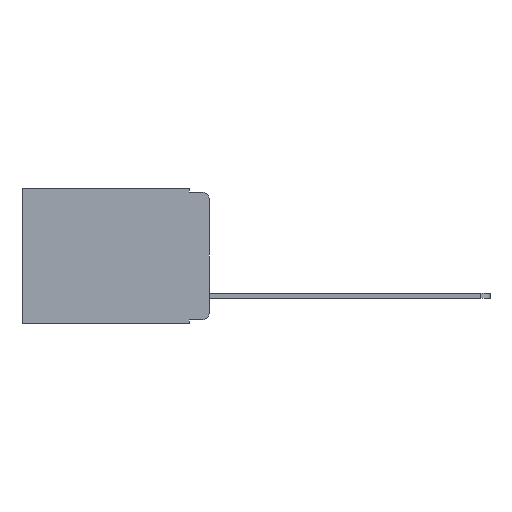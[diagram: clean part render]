
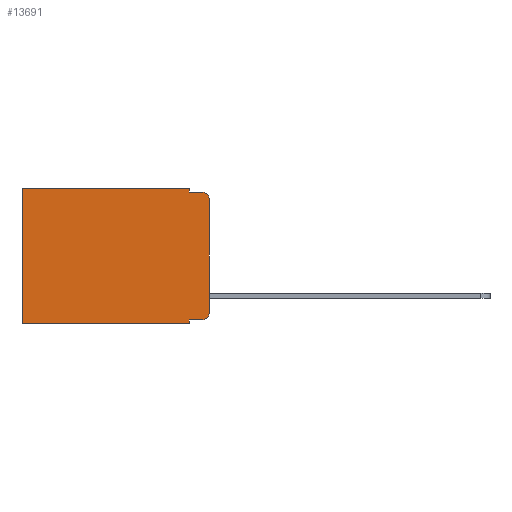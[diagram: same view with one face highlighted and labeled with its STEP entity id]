
A CAD part, left-side view. The second image highlights one B-rep face of the part: STEP entity #13691.
In plain terms, the highlighted planar face has unit normal (-1, 0, 0).
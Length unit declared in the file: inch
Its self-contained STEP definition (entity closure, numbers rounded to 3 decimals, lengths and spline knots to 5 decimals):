
#201 = DIRECTION ( 'NONE',  ( 0., 1., 0. ) ) ;
#272 = ORIENTED_EDGE ( 'NONE', *, *, #9066, .F. ) ;
#332 = CIRCLE ( 'NONE', #11500, 0.02 ) ;
#483 = ORIENTED_EDGE ( 'NONE', *, *, #6219, .T. ) ;
#559 = DIRECTION ( 'NONE',  ( 0., 0., -1. ) ) ;
#940 = CARTESIAN_POINT ( 'NONE',  ( 0.298, 0.051, -0.333 ) ) ;
#956 = CARTESIAN_POINT ( 'NONE',  ( 0.298, 0.051, 0. ) ) ;
#1117 = ORIENTED_EDGE ( 'NONE', *, *, #10961, .T. ) ;
#1229 = EDGE_CURVE ( 'NONE', #6926, #6484, #13971, .T. ) ;
#1267 = ORIENTED_EDGE ( 'NONE', *, *, #7857, .F. ) ;
#1395 = LINE ( 'NONE', #8242, #12024 ) ;
#1463 = VERTEX_POINT ( 'NONE', #2653 ) ;
#1621 = CARTESIAN_POINT ( 'NONE',  ( 0.298, 0., 0. ) ) ;
#1997 = CARTESIAN_POINT ( 'NONE',  ( 0.298, 0.473, 0. ) ) ;
#2028 = EDGE_LOOP ( 'NONE', ( #5095, #5801, #4200, #4830, #11334, #1117, #272, #1267, #5888, #483 ) ) ;
#2122 = VERTEX_POINT ( 'NONE', #2125 ) ;
#2125 = CARTESIAN_POINT ( 'NONE',  ( 0.298, 0., -0.03 ) ) ;
#2170 = VERTEX_POINT ( 'NONE', #4646 ) ;
#2208 = AXIS2_PLACEMENT_3D ( 'NONE', #11327, #4091, #12446 ) ;
#2275 = CARTESIAN_POINT ( 'NONE',  ( 0.298, 0.051, 0. ) ) ;
#2415 = LINE ( 'NONE', #15195, #8779 ) ;
#2466 = VECTOR ( 'NONE', #9824, 39.37008 ) ;
#2653 = CARTESIAN_POINT ( 'NONE',  ( 0.298, 0., -0.313 ) ) ;
#2771 = VERTEX_POINT ( 'NONE', #940 ) ;
#3162 = LINE ( 'NONE', #1621, #15330 ) ;
#4059 = VERTEX_POINT ( 'NONE', #7688 ) ;
#4091 = DIRECTION ( 'NONE',  ( -1., 0., 0. ) ) ;
#4178 = VERTEX_POINT ( 'NONE', #11527 ) ;
#4200 = ORIENTED_EDGE ( 'NONE', *, *, #12445, .F. ) ;
#4646 = CARTESIAN_POINT ( 'NONE',  ( 0.298, 0.02, -0.333 ) ) ;
#4824 = VECTOR ( 'NONE', #5585, 39.37008 ) ;
#4830 = ORIENTED_EDGE ( 'NONE', *, *, #11712, .F. ) ;
#4831 = LINE ( 'NONE', #1997, #14506 ) ;
#5095 = ORIENTED_EDGE ( 'NONE', *, *, #11428, .F. ) ;
#5585 = DIRECTION ( 'NONE',  ( 0., -1., 0. ) ) ;
#5801 = ORIENTED_EDGE ( 'NONE', *, *, #14666, .T. ) ;
#5848 = PLANE ( 'NONE',  #13890 ) ;
#5888 = ORIENTED_EDGE ( 'NONE', *, *, #7023, .T. ) ;
#5904 = CARTESIAN_POINT ( 'NONE',  ( 0.298, 0., 0. ) ) ;
#5924 = VERTEX_POINT ( 'NONE', #10656 ) ;
#6032 = VECTOR ( 'NONE', #12068, 39.37008 ) ;
#6219 = EDGE_CURVE ( 'NONE', #2170, #1463, #332, .T. ) ;
#6484 = VERTEX_POINT ( 'NONE', #10103 ) ;
#6793 = LINE ( 'NONE', #956, #6032 ) ;
#6926 = VERTEX_POINT ( 'NONE', #10390 ) ;
#7023 = EDGE_CURVE ( 'NONE', #2771, #2170, #1395, .T. ) ;
#7277 = DIRECTION ( 'NONE',  ( 0., 1., 0. ) ) ;
#7688 = CARTESIAN_POINT ( 'NONE',  ( 0.298, 0.02, -0.01 ) ) ;
#7776 = CARTESIAN_POINT ( 'NONE',  ( 0.298, 0.02, -0.313 ) ) ;
#7857 = EDGE_CURVE ( 'NONE', #2771, #14111, #11846, .T. ) ;
#8067 = DIRECTION ( 'NONE',  ( 0., 0., -1. ) ) ;
#8242 = CARTESIAN_POINT ( 'NONE',  ( 0.298, 0.051, -0.333 ) ) ;
#8344 = DIRECTION ( 'NONE',  ( 1., 0., 0. ) ) ;
#8779 = VECTOR ( 'NONE', #7277, 39.37008 ) ;
#9066 = EDGE_CURVE ( 'NONE', #14111, #4178, #2415, .T. ) ;
#9176 = CARTESIAN_POINT ( 'NONE',  ( 0.298, 0.051, -0.01 ) ) ;
#9586 = DIRECTION ( 'NONE',  ( 0., 0., -1. ) ) ;
#9824 = DIRECTION ( 'NONE',  ( 0., 0., -1. ) ) ;
#10103 = CARTESIAN_POINT ( 'NONE',  ( 0.298, 0.473, 0. ) ) ;
#10276 = CARTESIAN_POINT ( 'NONE',  ( 0.298, 0.051, -0.343 ) ) ;
#10390 = CARTESIAN_POINT ( 'NONE',  ( 0.298, 0.051, 0. ) ) ;
#10656 = CARTESIAN_POINT ( 'NONE',  ( 0.298, 0.051, -0.01 ) ) ;
#10703 = DIRECTION ( 'NONE',  ( 0., 0., -1. ) ) ;
#10812 = CIRCLE ( 'NONE', #2208, 0.02 ) ;
#10920 = DIRECTION ( 'NONE',  ( -1., 0., 0. ) ) ;
#10961 = EDGE_CURVE ( 'NONE', #6484, #4178, #4831, .T. ) ;
#11034 = VECTOR ( 'NONE', #201, 39.37008 ) ;
#11205 = LINE ( 'NONE', #9176, #4824 ) ;
#11327 = CARTESIAN_POINT ( 'NONE',  ( 0.298, 0.02, -0.03 ) ) ;
#11334 = ORIENTED_EDGE ( 'NONE', *, *, #1229, .T. ) ;
#11428 = EDGE_CURVE ( 'NONE', #2122, #1463, #3162, .T. ) ;
#11500 = AXIS2_PLACEMENT_3D ( 'NONE', #7776, #10920, #10703 ) ;
#11527 = CARTESIAN_POINT ( 'NONE',  ( 0.298, 0.473, -0.343 ) ) ;
#11657 = CARTESIAN_POINT ( 'NONE',  ( 0.298, 0., 0. ) ) ;
#11712 = EDGE_CURVE ( 'NONE', #6926, #5924, #6793, .T. ) ;
#11846 = LINE ( 'NONE', #2275, #2466 ) ;
#12024 = VECTOR ( 'NONE', #14968, 39.37008 ) ;
#12068 = DIRECTION ( 'NONE',  ( 0., 0., -1. ) ) ;
#12445 = EDGE_CURVE ( 'NONE', #5924, #4059, #11205, .T. ) ;
#12446 = DIRECTION ( 'NONE',  ( 0., 0., -1. ) ) ;
#13603 = FACE_OUTER_BOUND ( 'NONE', #2028, .T. ) ;
#13691 = ADVANCED_FACE ( 'NONE', ( #13603 ), #5848, .F. ) ;
#13890 = AXIS2_PLACEMENT_3D ( 'NONE', #5904, #8344, #559 ) ;
#13971 = LINE ( 'NONE', #11657, #11034 ) ;
#14111 = VERTEX_POINT ( 'NONE', #10276 ) ;
#14506 = VECTOR ( 'NONE', #9586, 39.37008 ) ;
#14666 = EDGE_CURVE ( 'NONE', #2122, #4059, #10812, .T. ) ;
#14968 = DIRECTION ( 'NONE',  ( 0., -1., 0. ) ) ;
#15195 = CARTESIAN_POINT ( 'NONE',  ( 0.298, 0., -0.343 ) ) ;
#15330 = VECTOR ( 'NONE', #8067, 39.37008 ) ;
